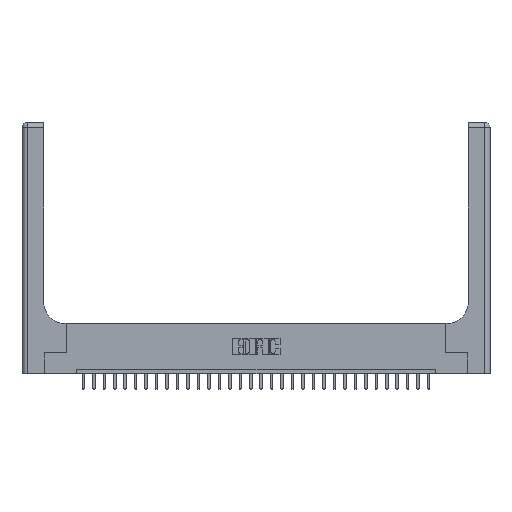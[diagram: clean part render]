
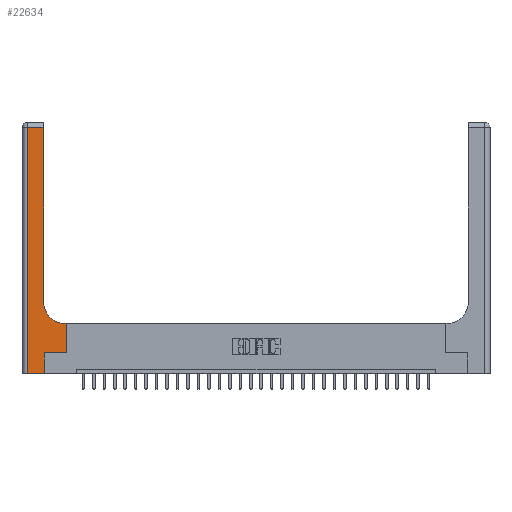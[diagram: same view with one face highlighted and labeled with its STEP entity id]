
A CAD part, top view. The second image highlights one B-rep face of the part: STEP entity #22634.
In plain terms, the highlighted planar face has unit normal (0, 0, 1).
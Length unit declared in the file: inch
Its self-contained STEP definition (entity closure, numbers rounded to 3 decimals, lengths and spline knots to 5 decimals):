
#406 = LINE ( 'NONE', #8753, #9928 ) ;
#528 = AXIS2_PLACEMENT_3D ( 'NONE', #10894, #23875, #11327 ) ;
#602 = ORIENTED_EDGE ( 'NONE', *, *, #8091, .T. ) ;
#929 = VECTOR ( 'NONE', #19519, 39.37008 ) ;
#1081 = DIRECTION ( 'NONE',  ( -1., 0., 0. ) ) ;
#1246 = ORIENTED_EDGE ( 'NONE', *, *, #24445, .T. ) ;
#1356 = EDGE_CURVE ( 'NONE', #3831, #19570, #2928, .T. ) ;
#2011 = AXIS2_PLACEMENT_3D ( 'NONE', #5043, #9527, #26470 ) ;
#2403 = DIRECTION ( 'NONE',  ( -1., 0., 0. ) ) ;
#2477 = CARTESIAN_POINT ( 'NONE',  ( 0.26, 0.85, 0.37 ) ) ;
#2928 = LINE ( 'NONE', #9263, #3589 ) ;
#3197 = CARTESIAN_POINT ( 'NONE',  ( 0., 0., 0.37 ) ) ;
#3589 = VECTOR ( 'NONE', #1081, 39.37008 ) ;
#3731 = VERTEX_POINT ( 'NONE', #21139 ) ;
#3831 = VERTEX_POINT ( 'NONE', #24358 ) ;
#4175 = CARTESIAN_POINT ( 'NONE',  ( 0.528, 0.25, 0.37 ) ) ;
#4338 = DIRECTION ( 'NONE',  ( 1., 0., 0. ) ) ;
#4354 = ORIENTED_EDGE ( 'NONE', *, *, #25508, .T. ) ;
#4388 = VECTOR ( 'NONE', #4338, 39.37008 ) ;
#4624 = EDGE_CURVE ( 'NONE', #24311, #3731, #23873, .T. ) ;
#4760 = CARTESIAN_POINT ( 'NONE',  ( 0.51, 0.6, 0.37 ) ) ;
#5043 = CARTESIAN_POINT ( 'NONE',  ( 0., 3., 0.37 ) ) ;
#5082 = EDGE_LOOP ( 'NONE', ( #17267, #17124, #12149, #602, #11446, #15209, #1246, #12332, #4354 ) ) ;
#6308 = CARTESIAN_POINT ( 'NONE',  ( 0.265, 0.25, 0.37 ) ) ;
#6967 = CARTESIAN_POINT ( 'NONE',  ( 0.06, 3., 0.37 ) ) ;
#7064 = EDGE_CURVE ( 'NONE', #26994, #27353, #26885, .T. ) ;
#8091 = EDGE_CURVE ( 'NONE', #3731, #15234, #20409, .T. ) ;
#8753 = CARTESIAN_POINT ( 'NONE',  ( 0.265, 0., 0.37 ) ) ;
#8912 = CARTESIAN_POINT ( 'NONE',  ( 0.26, 2.94, 0.37 ) ) ;
#9203 = VECTOR ( 'NONE', #2403, 39.37008 ) ;
#9263 = CARTESIAN_POINT ( 'NONE',  ( 0.26, 0.6, 0.37 ) ) ;
#9527 = DIRECTION ( 'NONE',  ( 0., 0., -1. ) ) ;
#9775 = VERTEX_POINT ( 'NONE', #23744 ) ;
#9928 = VECTOR ( 'NONE', #15051, 39.37008 ) ;
#10894 = CARTESIAN_POINT ( 'NONE',  ( 0.51, 0.85, 0.37 ) ) ;
#11327 = DIRECTION ( 'NONE',  ( 1., 0., 0. ) ) ;
#11446 = ORIENTED_EDGE ( 'NONE', *, *, #15780, .T. ) ;
#12149 = ORIENTED_EDGE ( 'NONE', *, *, #4624, .T. ) ;
#12182 = EDGE_CURVE ( 'NONE', #9775, #13894, #20728, .T. ) ;
#12332 = ORIENTED_EDGE ( 'NONE', *, *, #1356, .T. ) ;
#12974 = LINE ( 'NONE', #13533, #9203 ) ;
#13533 = CARTESIAN_POINT ( 'NONE',  ( 0., 2.94, 0.37 ) ) ;
#13746 = DIRECTION ( 'NONE',  ( 0., 1., 0. ) ) ;
#13894 = VERTEX_POINT ( 'NONE', #4175 ) ;
#14031 = VECTOR ( 'NONE', #24009, 39.37008 ) ;
#15051 = DIRECTION ( 'NONE',  ( 0., 1., 0. ) ) ;
#15209 = ORIENTED_EDGE ( 'NONE', *, *, #12182, .T. ) ;
#15234 = VERTEX_POINT ( 'NONE', #23590 ) ;
#15595 = FACE_OUTER_BOUND ( 'NONE', #5082, .T. ) ;
#15780 = EDGE_CURVE ( 'NONE', #15234, #9775, #406, .T. ) ;
#17124 = ORIENTED_EDGE ( 'NONE', *, *, #22115, .T. ) ;
#17246 = CARTESIAN_POINT ( 'NONE',  ( 0.528, 0.25, 0.37 ) ) ;
#17267 = ORIENTED_EDGE ( 'NONE', *, *, #7064, .T. ) ;
#18013 = PLANE ( 'NONE',  #2011 ) ;
#18279 = CARTESIAN_POINT ( 'NONE',  ( 0.26, 3., 0.37 ) ) ;
#19480 = VECTOR ( 'NONE', #13746, 39.37008 ) ;
#19519 = DIRECTION ( 'NONE',  ( 0., 1., 0. ) ) ;
#19570 = VERTEX_POINT ( 'NONE', #4760 ) ;
#19791 = LINE ( 'NONE', #17246, #929 ) ;
#20409 = LINE ( 'NONE', #3197, #25264 ) ;
#20728 = LINE ( 'NONE', #6308, #4388 ) ;
#21139 = CARTESIAN_POINT ( 'NONE',  ( 0.06, 0., 0.37 ) ) ;
#22115 = EDGE_CURVE ( 'NONE', #27353, #24311, #12974, .T. ) ;
#22361 = DIRECTION ( 'NONE',  ( 1., 0., 0. ) ) ;
#22634 = ADVANCED_FACE ( 'NONE', ( #15595 ), #18013, .F. ) ;
#23322 = CARTESIAN_POINT ( 'NONE',  ( 0.06, 2.94, 0.37 ) ) ;
#23590 = CARTESIAN_POINT ( 'NONE',  ( 0.265, 0., 0.37 ) ) ;
#23744 = CARTESIAN_POINT ( 'NONE',  ( 0.265, 0.25, 0.37 ) ) ;
#23873 = LINE ( 'NONE', #6967, #14031 ) ;
#23875 = DIRECTION ( 'NONE',  ( 0., 0., -1. ) ) ;
#24009 = DIRECTION ( 'NONE',  ( 0., -1., 0. ) ) ;
#24311 = VERTEX_POINT ( 'NONE', #23322 ) ;
#24358 = CARTESIAN_POINT ( 'NONE',  ( 0.528, 0.6, 0.37 ) ) ;
#24445 = EDGE_CURVE ( 'NONE', #13894, #3831, #19791, .T. ) ;
#25264 = VECTOR ( 'NONE', #22361, 39.37008 ) ;
#25308 = CIRCLE ( 'NONE', #528, 0.25 ) ;
#25508 = EDGE_CURVE ( 'NONE', #19570, #26994, #25308, .T. ) ;
#26470 = DIRECTION ( 'NONE',  ( -1., 0., 0. ) ) ;
#26885 = LINE ( 'NONE', #18279, #19480 ) ;
#26994 = VERTEX_POINT ( 'NONE', #2477 ) ;
#27353 = VERTEX_POINT ( 'NONE', #8912 ) ;
